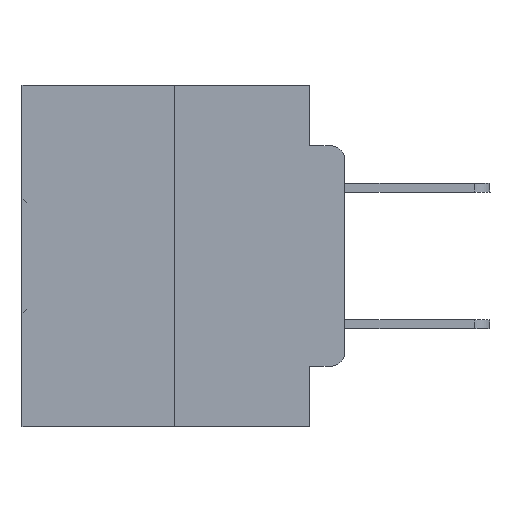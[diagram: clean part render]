
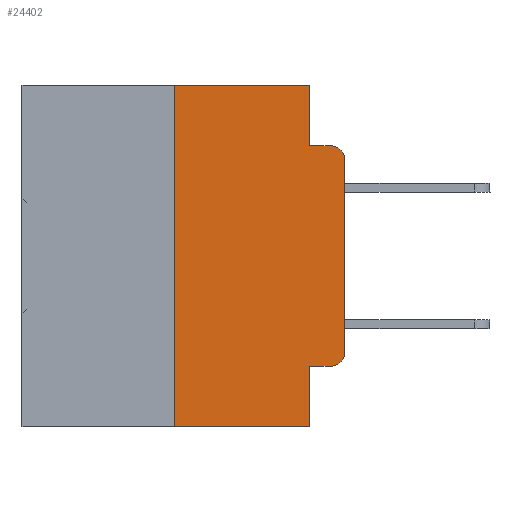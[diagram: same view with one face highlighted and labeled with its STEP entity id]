
A CAD part, left-side view. The second image highlights one B-rep face of the part: STEP entity #24402.
In plain terms, the highlighted planar face has unit normal (-1, 0, 0).
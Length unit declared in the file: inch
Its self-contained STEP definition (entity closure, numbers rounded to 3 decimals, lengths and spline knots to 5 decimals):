
#1271 = LINE ( 'NONE', #10966, #18147 ) ;
#1571 = DIRECTION ( 'NONE',  ( 0., 0., 1. ) ) ;
#2026 = EDGE_CURVE ( 'NONE', #29856, #2595, #29740, .T. ) ;
#2032 = CARTESIAN_POINT ( 'NONE',  ( 0., 0.051, -0.4115 ) ) ;
#2340 = EDGE_CURVE ( 'NONE', #2595, #17322, #26423, .T. ) ;
#2426 = CARTESIAN_POINT ( 'NONE',  ( 0., 0.25, 0. ) ) ;
#2429 = CARTESIAN_POINT ( 'NONE',  ( 0., 0.473, 0. ) ) ;
#2448 = VECTOR ( 'NONE', #26917, 39.37008 ) ;
#2485 = CARTESIAN_POINT ( 'NONE',  ( 0., 0.051, -0.0885 ) ) ;
#2595 = VERTEX_POINT ( 'NONE', #14704 ) ;
#3979 = VERTEX_POINT ( 'NONE', #2032 ) ;
#4318 = EDGE_CURVE ( 'NONE', #3979, #27042, #7892, .T. ) ;
#4443 = AXIS2_PLACEMENT_3D ( 'NONE', #2429, #28705, #26412 ) ;
#5386 = LINE ( 'NONE', #31990, #17314 ) ;
#5944 = CARTESIAN_POINT ( 'NONE',  ( 0., 0.051, 0. ) ) ;
#5953 = VECTOR ( 'NONE', #14392, 39.37008 ) ;
#6495 = ORIENTED_EDGE ( 'NONE', *, *, #2340, .T. ) ;
#6787 = AXIS2_PLACEMENT_3D ( 'NONE', #8631, #32519, #32640 ) ;
#6863 = EDGE_CURVE ( 'NONE', #17085, #9674, #5386, .T. ) ;
#7575 = VERTEX_POINT ( 'NONE', #2426 ) ;
#7892 = LINE ( 'NONE', #16658, #17385 ) ;
#8027 = CARTESIAN_POINT ( 'NONE',  ( 0., 0.051, 0. ) ) ;
#8256 = LINE ( 'NONE', #2485, #15678 ) ;
#8631 = CARTESIAN_POINT ( 'NONE',  ( 0., 0.02, -0.1085 ) ) ;
#9199 = CARTESIAN_POINT ( 'NONE',  ( 0., 0.25, -0.5 ) ) ;
#9226 = CARTESIAN_POINT ( 'NONE',  ( 0., 0.051, -0.0885 ) ) ;
#9674 = VERTEX_POINT ( 'NONE', #11668 ) ;
#9968 = VERTEX_POINT ( 'NONE', #8027 ) ;
#10447 = ORIENTED_EDGE ( 'NONE', *, *, #15540, .F. ) ;
#10646 = PLANE ( 'NONE',  #4443 ) ;
#10876 = DIRECTION ( 'NONE',  ( -1., 0., 0. ) ) ;
#10966 = CARTESIAN_POINT ( 'NONE',  ( 0., 0.051, 0. ) ) ;
#11668 = CARTESIAN_POINT ( 'NONE',  ( 0., 0.051, -0.5 ) ) ;
#11979 = LINE ( 'NONE', #5944, #2448 ) ;
#12967 = CARTESIAN_POINT ( 'NONE',  ( 0., 0.02, -0.0885 ) ) ;
#13376 = DIRECTION ( 'NONE',  ( 0., 0., -1. ) ) ;
#14164 = ORIENTED_EDGE ( 'NONE', *, *, #32515, .F. ) ;
#14392 = DIRECTION ( 'NONE',  ( 0., -1., 0. ) ) ;
#14691 = CIRCLE ( 'NONE', #32053, 0.02 ) ;
#14704 = CARTESIAN_POINT ( 'NONE',  ( 0., 0., -0.1085 ) ) ;
#15540 = EDGE_CURVE ( 'NONE', #17085, #7575, #17292, .T. ) ;
#15678 = VECTOR ( 'NONE', #31707, 39.37008 ) ;
#15779 = ORIENTED_EDGE ( 'NONE', *, *, #6863, .T. ) ;
#16658 = CARTESIAN_POINT ( 'NONE',  ( 0., 0.051, -0.4115 ) ) ;
#17085 = VERTEX_POINT ( 'NONE', #9199 ) ;
#17292 = LINE ( 'NONE', #33772, #29940 ) ;
#17314 = VECTOR ( 'NONE', #19115, 39.37008 ) ;
#17322 = VERTEX_POINT ( 'NONE', #12967 ) ;
#17338 = CARTESIAN_POINT ( 'NONE',  ( 0., 0., 0. ) ) ;
#17377 = CARTESIAN_POINT ( 'NONE',  ( 0., 0.473, 0. ) ) ;
#17385 = VECTOR ( 'NONE', #19271, 39.37008 ) ;
#17509 = VECTOR ( 'NONE', #1571, 39.37008 ) ;
#18147 = VECTOR ( 'NONE', #13376, 39.37008 ) ;
#18678 = DIRECTION ( 'NONE',  ( 0., 0., -1. ) ) ;
#19115 = DIRECTION ( 'NONE',  ( 0., -1., 0. ) ) ;
#19271 = DIRECTION ( 'NONE',  ( 0., -1., 0. ) ) ;
#19665 = ORIENTED_EDGE ( 'NONE', *, *, #29949, .F. ) ;
#19726 = ORIENTED_EDGE ( 'NONE', *, *, #20645, .F. ) ;
#20068 = EDGE_CURVE ( 'NONE', #9968, #29055, #1271, .T. ) ;
#20645 = EDGE_CURVE ( 'NONE', #29055, #17322, #8256, .T. ) ;
#22014 = ORIENTED_EDGE ( 'NONE', *, *, #22418, .T. ) ;
#22319 = ORIENTED_EDGE ( 'NONE', *, *, #20068, .F. ) ;
#22418 = EDGE_CURVE ( 'NONE', #27042, #29856, #14691, .T. ) ;
#23344 = CARTESIAN_POINT ( 'NONE',  ( 0., 0., -0.3915 ) ) ;
#23980 = LINE ( 'NONE', #17377, #5953 ) ;
#24402 = ADVANCED_FACE ( 'NONE', ( #27251 ), #10646, .F. ) ;
#24654 = ORIENTED_EDGE ( 'NONE', *, *, #4318, .T. ) ;
#26412 = DIRECTION ( 'NONE',  ( 0., 0., -1. ) ) ;
#26423 = CIRCLE ( 'NONE', #6787, 0.02 ) ;
#26520 = CARTESIAN_POINT ( 'NONE',  ( 0., 0.02, -0.4115 ) ) ;
#26917 = DIRECTION ( 'NONE',  ( 0., 0., -1. ) ) ;
#27042 = VERTEX_POINT ( 'NONE', #26520 ) ;
#27251 = FACE_OUTER_BOUND ( 'NONE', #32390, .T. ) ;
#28705 = DIRECTION ( 'NONE',  ( 1., 0., 0. ) ) ;
#28741 = DIRECTION ( 'NONE',  ( 0., 0., 1. ) ) ;
#29055 = VERTEX_POINT ( 'NONE', #9226 ) ;
#29285 = CARTESIAN_POINT ( 'NONE',  ( 0., 0.02, -0.3915 ) ) ;
#29740 = LINE ( 'NONE', #17338, #17509 ) ;
#29856 = VERTEX_POINT ( 'NONE', #23344 ) ;
#29940 = VECTOR ( 'NONE', #28741, 39.37008 ) ;
#29949 = EDGE_CURVE ( 'NONE', #3979, #9674, #11979, .T. ) ;
#31465 = ORIENTED_EDGE ( 'NONE', *, *, #2026, .T. ) ;
#31707 = DIRECTION ( 'NONE',  ( 0., -1., 0. ) ) ;
#31990 = CARTESIAN_POINT ( 'NONE',  ( 0., 0.473, -0.5 ) ) ;
#32053 = AXIS2_PLACEMENT_3D ( 'NONE', #29285, #10876, #18678 ) ;
#32390 = EDGE_LOOP ( 'NONE', ( #31465, #6495, #19726, #22319, #14164, #10447, #15779, #19665, #24654, #22014 ) ) ;
#32515 = EDGE_CURVE ( 'NONE', #7575, #9968, #23980, .T. ) ;
#32519 = DIRECTION ( 'NONE',  ( -1., 0., 0. ) ) ;
#32640 = DIRECTION ( 'NONE',  ( 0., 0., -1. ) ) ;
#33772 = CARTESIAN_POINT ( 'NONE',  ( 0., 0.25, 0. ) ) ;
